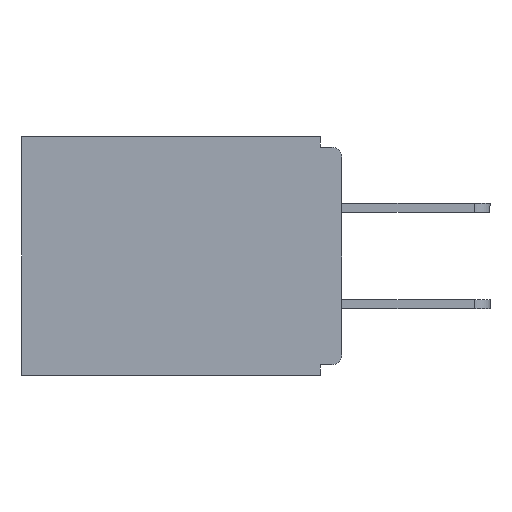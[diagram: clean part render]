
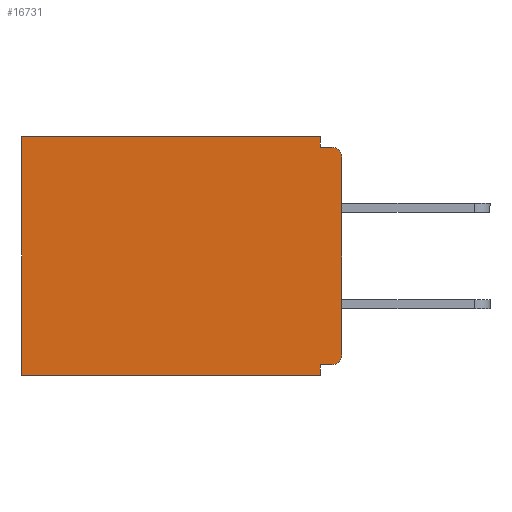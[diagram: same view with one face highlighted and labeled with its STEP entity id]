
A CAD part, left-side view. The second image highlights one B-rep face of the part: STEP entity #16731.
In plain terms, the highlighted planar face has unit normal (-1, 0, 0).
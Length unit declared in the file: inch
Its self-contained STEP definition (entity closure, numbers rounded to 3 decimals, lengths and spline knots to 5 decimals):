
#40 = VERTEX_POINT ( 'NONE', #11645 ) ;
#70 = DIRECTION ( 'NONE',  ( 0., 0., -1. ) ) ;
#133 = EDGE_CURVE ( 'NONE', #7526, #17716, #16327, .T. ) ;
#564 = CARTESIAN_POINT ( 'NONE',  ( 0.298, 0., -0.343 ) ) ;
#706 = LINE ( 'NONE', #2761, #22483 ) ;
#1007 = ORIENTED_EDGE ( 'NONE', *, *, #25372, .F. ) ;
#1083 = VECTOR ( 'NONE', #7595, 39.37008 ) ;
#1597 = LINE ( 'NONE', #8891, #22683 ) ;
#1770 = VERTEX_POINT ( 'NONE', #13383 ) ;
#1796 = CARTESIAN_POINT ( 'NONE',  ( 0.298, 0., -0.015 ) ) ;
#1815 = DIRECTION ( 'NONE',  ( -1., 0., 0. ) ) ;
#1873 = CARTESIAN_POINT ( 'NONE',  ( 0.298, 0.015, -0.015 ) ) ;
#2476 = EDGE_CURVE ( 'NONE', #24795, #12343, #6026, .T. ) ;
#2646 = FACE_OUTER_BOUND ( 'NONE', #10993, .T. ) ;
#2761 = CARTESIAN_POINT ( 'NONE',  ( 0.298, 0., -0.328 ) ) ;
#3095 = DIRECTION ( 'NONE',  ( 0., 0., -1. ) ) ;
#4403 = CARTESIAN_POINT ( 'NONE',  ( 0.298, 0., -0.313 ) ) ;
#4432 = VECTOR ( 'NONE', #26718, 39.37008 ) ;
#4866 = CIRCLE ( 'NONE', #14013, 0.015 ) ;
#5044 = CARTESIAN_POINT ( 'NONE',  ( 0.298, 0.031, -0.343 ) ) ;
#5102 = DIRECTION ( 'NONE',  ( 0., 1., 0. ) ) ;
#5205 = ORIENTED_EDGE ( 'NONE', *, *, #19407, .F. ) ;
#5930 = EDGE_CURVE ( 'NONE', #12174, #25038, #4866, .T. ) ;
#6026 = LINE ( 'NONE', #564, #8896 ) ;
#6369 = ORIENTED_EDGE ( 'NONE', *, *, #26801, .T. ) ;
#6460 = LINE ( 'NONE', #16165, #14525 ) ;
#6485 = EDGE_CURVE ( 'NONE', #8643, #12343, #6460, .T. ) ;
#6616 = LINE ( 'NONE', #17692, #1083 ) ;
#6876 = ORIENTED_EDGE ( 'NONE', *, *, #8205, .F. ) ;
#7526 = VERTEX_POINT ( 'NONE', #15518 ) ;
#7595 = DIRECTION ( 'NONE',  ( 0., 1., 0. ) ) ;
#7925 = LINE ( 'NONE', #15441, #25383 ) ;
#7988 = ORIENTED_EDGE ( 'NONE', *, *, #5930, .T. ) ;
#8205 = EDGE_CURVE ( 'NONE', #12174, #17716, #1597, .T. ) ;
#8340 = ORIENTED_EDGE ( 'NONE', *, *, #26079, .F. ) ;
#8643 = VERTEX_POINT ( 'NONE', #9190 ) ;
#8891 = CARTESIAN_POINT ( 'NONE',  ( 0.298, 0., 0. ) ) ;
#8896 = VECTOR ( 'NONE', #25467, 39.37008 ) ;
#9190 = CARTESIAN_POINT ( 'NONE',  ( 0.298, 0.46, 0. ) ) ;
#9618 = ORIENTED_EDGE ( 'NONE', *, *, #2476, .F. ) ;
#10993 = EDGE_LOOP ( 'NONE', ( #7988, #5205, #24559, #6369, #25607, #9618, #8340, #1007, #13257, #6876 ) ) ;
#11645 = CARTESIAN_POINT ( 'NONE',  ( 0.298, 0.031, -0.328 ) ) ;
#12046 = DIRECTION ( 'NONE',  ( 0., 0., -1. ) ) ;
#12174 = VERTEX_POINT ( 'NONE', #17199 ) ;
#12343 = VERTEX_POINT ( 'NONE', #19637 ) ;
#12650 = VECTOR ( 'NONE', #70, 39.37008 ) ;
#12935 = DIRECTION ( 'NONE',  ( 0., 0., -1. ) ) ;
#13257 = ORIENTED_EDGE ( 'NONE', *, *, #133, .T. ) ;
#13383 = CARTESIAN_POINT ( 'NONE',  ( 0.298, 0.031, -0.015 ) ) ;
#13771 = DIRECTION ( 'NONE',  ( 0., 0., -1. ) ) ;
#14013 = AXIS2_PLACEMENT_3D ( 'NONE', #20245, #26241, #13771 ) ;
#14179 = CARTESIAN_POINT ( 'NONE',  ( 0.298, 0.015, -0.313 ) ) ;
#14525 = VECTOR ( 'NONE', #22280, 39.37008 ) ;
#15441 = CARTESIAN_POINT ( 'NONE',  ( 0.298, 0.031, -0.343 ) ) ;
#15518 = CARTESIAN_POINT ( 'NONE',  ( 0.298, 0.015, -0.328 ) ) ;
#16165 = CARTESIAN_POINT ( 'NONE',  ( 0.298, 0.46, 0. ) ) ;
#16327 = CIRCLE ( 'NONE', #25760, 0.015 ) ;
#16329 = CARTESIAN_POINT ( 'NONE',  ( 0.298, 0.031, -0.343 ) ) ;
#16731 = ADVANCED_FACE ( 'NONE', ( #2646 ), #24861, .F. ) ;
#17199 = CARTESIAN_POINT ( 'NONE',  ( 0.298, 0., -0.03 ) ) ;
#17692 = CARTESIAN_POINT ( 'NONE',  ( 0.298, 0., 0. ) ) ;
#17716 = VERTEX_POINT ( 'NONE', #4403 ) ;
#18189 = AXIS2_PLACEMENT_3D ( 'NONE', #24687, #20428, #12046 ) ;
#18661 = LINE ( 'NONE', #1796, #4432 ) ;
#19000 = CARTESIAN_POINT ( 'NONE',  ( 0.298, 0.031, 0. ) ) ;
#19407 = EDGE_CURVE ( 'NONE', #1770, #25038, #18661, .T. ) ;
#19637 = CARTESIAN_POINT ( 'NONE',  ( 0.298, 0.46, -0.343 ) ) ;
#20245 = CARTESIAN_POINT ( 'NONE',  ( 0.298, 0.015, -0.03 ) ) ;
#20428 = DIRECTION ( 'NONE',  ( 1., 0., 0. ) ) ;
#22280 = DIRECTION ( 'NONE',  ( 0., 0., -1. ) ) ;
#22483 = VECTOR ( 'NONE', #5102, 39.37008 ) ;
#22683 = VECTOR ( 'NONE', #12935, 39.37008 ) ;
#24053 = LINE ( 'NONE', #16329, #12650 ) ;
#24481 = EDGE_CURVE ( 'NONE', #26709, #1770, #7925, .T. ) ;
#24559 = ORIENTED_EDGE ( 'NONE', *, *, #24481, .F. ) ;
#24653 = DIRECTION ( 'NONE',  ( 0., 0., -1. ) ) ;
#24687 = CARTESIAN_POINT ( 'NONE',  ( 0.298, 0., 0. ) ) ;
#24795 = VERTEX_POINT ( 'NONE', #5044 ) ;
#24861 = PLANE ( 'NONE',  #18189 ) ;
#25038 = VERTEX_POINT ( 'NONE', #1873 ) ;
#25372 = EDGE_CURVE ( 'NONE', #7526, #40, #706, .T. ) ;
#25383 = VECTOR ( 'NONE', #3095, 39.37008 ) ;
#25467 = DIRECTION ( 'NONE',  ( 0., 1., 0. ) ) ;
#25607 = ORIENTED_EDGE ( 'NONE', *, *, #6485, .T. ) ;
#25760 = AXIS2_PLACEMENT_3D ( 'NONE', #14179, #1815, #24653 ) ;
#26079 = EDGE_CURVE ( 'NONE', #40, #24795, #24053, .T. ) ;
#26241 = DIRECTION ( 'NONE',  ( -1., 0., 0. ) ) ;
#26709 = VERTEX_POINT ( 'NONE', #19000 ) ;
#26718 = DIRECTION ( 'NONE',  ( 0., -1., 0. ) ) ;
#26801 = EDGE_CURVE ( 'NONE', #26709, #8643, #6616, .T. ) ;
